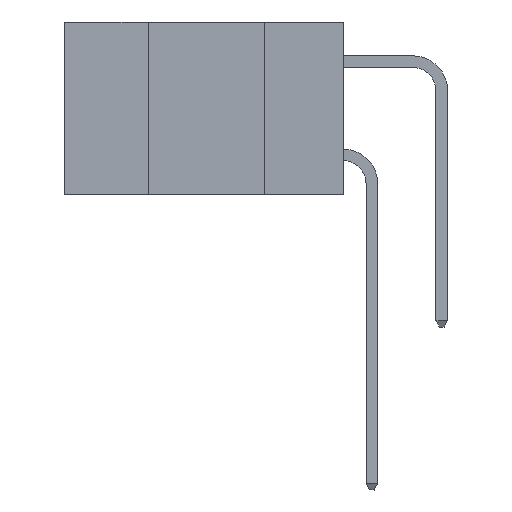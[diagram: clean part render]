
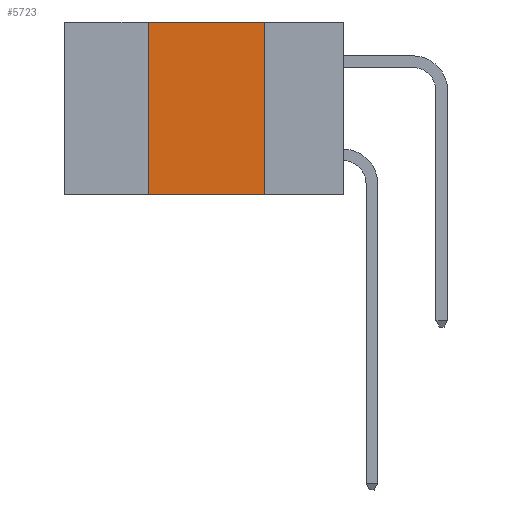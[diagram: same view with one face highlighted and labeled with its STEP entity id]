
A CAD part, left-side view. The second image highlights one B-rep face of the part: STEP entity #5723.
In plain terms, the highlighted planar face has unit normal (-1, 0, 0).
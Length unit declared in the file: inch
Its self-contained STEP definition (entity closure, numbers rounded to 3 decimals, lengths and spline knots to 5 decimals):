
#104 = CARTESIAN_POINT ( 'NONE',  ( 0., 0.6, 0. ) ) ;
#736 = ORIENTED_EDGE ( 'NONE', *, *, #2689, .F. ) ;
#799 = CARTESIAN_POINT ( 'NONE',  ( 0., 0.6, 0. ) ) ;
#1733 = EDGE_CURVE ( 'NONE', #8554, #9031, #10882, .T. ) ;
#1909 = EDGE_CURVE ( 'NONE', #10659, #15683, #4010, .T. ) ;
#1946 = ORIENTED_EDGE ( 'NONE', *, *, #16237, .T. ) ;
#2614 = CARTESIAN_POINT ( 'NONE',  ( 0., 0.42, -0.37 ) ) ;
#2689 = EDGE_CURVE ( 'NONE', #9031, #10659, #13111, .T. ) ;
#3346 = PLANE ( 'NONE',  #17173 ) ;
#4010 = LINE ( 'NONE', #16164, #14481 ) ;
#4297 = VECTOR ( 'NONE', #16367, 39.37008 ) ;
#4308 = CARTESIAN_POINT ( 'NONE',  ( 0., 0.6, -0.37 ) ) ;
#5723 = ADVANCED_FACE ( 'NONE', ( #13591 ), #3346, .F. ) ;
#6977 = DIRECTION ( 'NONE',  ( 0., 0., -1. ) ) ;
#7436 = ORIENTED_EDGE ( 'NONE', *, *, #1733, .F. ) ;
#8404 = DIRECTION ( 'NONE',  ( 0., -1., 0. ) ) ;
#8554 = VERTEX_POINT ( 'NONE', #2614 ) ;
#9031 = VERTEX_POINT ( 'NONE', #15858 ) ;
#10580 = LINE ( 'NONE', #4308, #4297 ) ;
#10586 = CARTESIAN_POINT ( 'NONE',  ( 0., 0.17, 0. ) ) ;
#10659 = VERTEX_POINT ( 'NONE', #10586 ) ;
#10882 = LINE ( 'NONE', #16860, #18495 ) ;
#13107 = VECTOR ( 'NONE', #8404, 39.37008 ) ;
#13111 = LINE ( 'NONE', #799, #13107 ) ;
#13591 = FACE_OUTER_BOUND ( 'NONE', #15250, .T. ) ;
#13681 = DIRECTION ( 'NONE',  ( 1., 0., 0. ) ) ;
#14481 = VECTOR ( 'NONE', #6977, 39.37008 ) ;
#15250 = EDGE_LOOP ( 'NONE', ( #16914, #736, #7436, #1946 ) ) ;
#15328 = DIRECTION ( 'NONE',  ( 0., 0., -1. ) ) ;
#15683 = VERTEX_POINT ( 'NONE', #17580 ) ;
#15858 = CARTESIAN_POINT ( 'NONE',  ( 0., 0.42, 0. ) ) ;
#16164 = CARTESIAN_POINT ( 'NONE',  ( 0., 0.17, -0.37 ) ) ;
#16237 = EDGE_CURVE ( 'NONE', #8554, #15683, #10580, .T. ) ;
#16367 = DIRECTION ( 'NONE',  ( 0., -1., 0. ) ) ;
#16860 = CARTESIAN_POINT ( 'NONE',  ( 0., 0.42, -0.37 ) ) ;
#16914 = ORIENTED_EDGE ( 'NONE', *, *, #1909, .F. ) ;
#17173 = AXIS2_PLACEMENT_3D ( 'NONE', #104, #13681, #15328 ) ;
#17580 = CARTESIAN_POINT ( 'NONE',  ( 0., 0.17, -0.37 ) ) ;
#18399 = DIRECTION ( 'NONE',  ( 0., 0., 1. ) ) ;
#18495 = VECTOR ( 'NONE', #18399, 39.37008 ) ;
